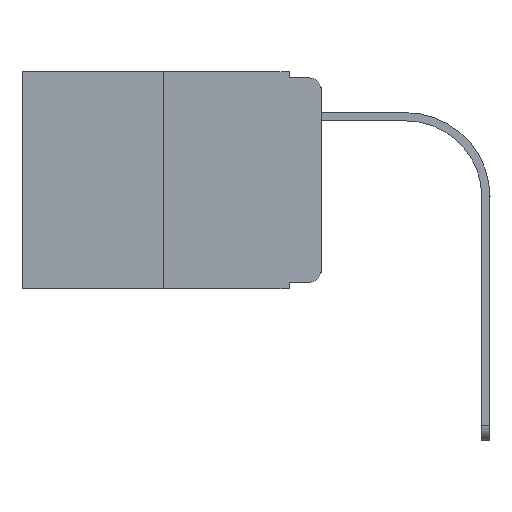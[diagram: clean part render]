
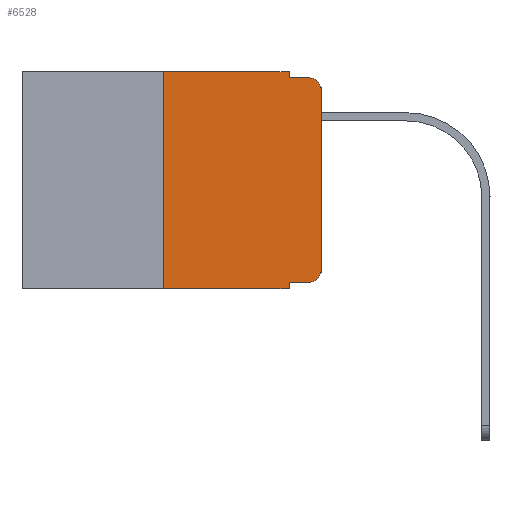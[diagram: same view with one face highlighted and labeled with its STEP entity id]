
A CAD part, left-side view. The second image highlights one B-rep face of the part: STEP entity #6528.
In plain terms, the highlighted planar face has unit normal (-1, 0, 0).
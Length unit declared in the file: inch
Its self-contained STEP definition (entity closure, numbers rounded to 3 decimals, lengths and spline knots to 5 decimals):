
#73 = CARTESIAN_POINT ( 'NONE',  ( 0., 0.051, 0. ) ) ;
#484 = LINE ( 'NONE', #7855, #7972 ) ;
#910 = CARTESIAN_POINT ( 'NONE',  ( 0., 0.25, 0. ) ) ;
#1019 = DIRECTION ( 'NONE',  ( 0., 0., -1. ) ) ;
#1084 = ORIENTED_EDGE ( 'NONE', *, *, #16197, .T. ) ;
#1193 = PLANE ( 'NONE',  #11289 ) ;
#1265 = VECTOR ( 'NONE', #6964, 39.37008 ) ;
#1766 = ORIENTED_EDGE ( 'NONE', *, *, #14694, .F. ) ;
#2194 = VECTOR ( 'NONE', #1019, 39.37008 ) ;
#2731 = VERTEX_POINT ( 'NONE', #16552 ) ;
#2794 = CARTESIAN_POINT ( 'NONE',  ( 0., 0.051, 0. ) ) ;
#3073 = EDGE_CURVE ( 'NONE', #6811, #2731, #14560, .T. ) ;
#3363 = AXIS2_PLACEMENT_3D ( 'NONE', #3949, #7374, #5882 ) ;
#3430 = CARTESIAN_POINT ( 'NONE',  ( 0., 0.473, 0. ) ) ;
#3626 = VECTOR ( 'NONE', #15949, 39.37008 ) ;
#3661 = DIRECTION ( 'NONE',  ( 0., -1., 0. ) ) ;
#3810 = CARTESIAN_POINT ( 'NONE',  ( 0., 0., 0. ) ) ;
#3916 = CARTESIAN_POINT ( 'NONE',  ( 0., 0.473, 0. ) ) ;
#3949 = CARTESIAN_POINT ( 'NONE',  ( 0., 0.02, -0.03 ) ) ;
#4098 = LINE ( 'NONE', #2794, #2194 ) ;
#4325 = DIRECTION ( 'NONE',  ( 0., 0., -1. ) ) ;
#4702 = ORIENTED_EDGE ( 'NONE', *, *, #12635, .T. ) ;
#4916 = LINE ( 'NONE', #3430, #10416 ) ;
#4945 = LINE ( 'NONE', #73, #10716 ) ;
#5126 = EDGE_CURVE ( 'NONE', #10448, #17928, #4098, .T. ) ;
#5464 = CARTESIAN_POINT ( 'NONE',  ( 0., 0.051, -0.01 ) ) ;
#5467 = LINE ( 'NONE', #16133, #7772 ) ;
#5882 = DIRECTION ( 'NONE',  ( 0., 0., -1. ) ) ;
#6190 = ORIENTED_EDGE ( 'NONE', *, *, #16955, .F. ) ;
#6506 = DIRECTION ( 'NONE',  ( 0., -1., 0. ) ) ;
#6528 = ADVANCED_FACE ( 'NONE', ( #8108 ), #1193, .F. ) ;
#6811 = VERTEX_POINT ( 'NONE', #9234 ) ;
#6950 = EDGE_CURVE ( 'NONE', #9740, #12576, #5467, .T. ) ;
#6964 = DIRECTION ( 'NONE',  ( 0., 0., 1. ) ) ;
#7374 = DIRECTION ( 'NONE',  ( -1., 0., 0. ) ) ;
#7514 = CARTESIAN_POINT ( 'NONE',  ( 0., 0.051, -0.343 ) ) ;
#7772 = VECTOR ( 'NONE', #17823, 39.37008 ) ;
#7838 = CIRCLE ( 'NONE', #3363, 0.02 ) ;
#7855 = CARTESIAN_POINT ( 'NONE',  ( 0., 0.051, -0.01 ) ) ;
#7972 = VECTOR ( 'NONE', #3661, 39.37008 ) ;
#8108 = FACE_OUTER_BOUND ( 'NONE', #16885, .T. ) ;
#8746 = DIRECTION ( 'NONE',  ( 0., -1., 0. ) ) ;
#8942 = CARTESIAN_POINT ( 'NONE',  ( 0., 0.051, 0. ) ) ;
#9223 = ORIENTED_EDGE ( 'NONE', *, *, #5126, .F. ) ;
#9234 = CARTESIAN_POINT ( 'NONE',  ( 0., 0.25, -0.343 ) ) ;
#9686 = ORIENTED_EDGE ( 'NONE', *, *, #18891, .T. ) ;
#9688 = ORIENTED_EDGE ( 'NONE', *, *, #3073, .F. ) ;
#9740 = VERTEX_POINT ( 'NONE', #16122 ) ;
#9807 = LINE ( 'NONE', #3810, #3626 ) ;
#10235 = VERTEX_POINT ( 'NONE', #16200 ) ;
#10416 = VECTOR ( 'NONE', #6506, 39.37008 ) ;
#10448 = VERTEX_POINT ( 'NONE', #8942 ) ;
#10490 = VERTEX_POINT ( 'NONE', #7514 ) ;
#10716 = VECTOR ( 'NONE', #13944, 39.37008 ) ;
#11289 = AXIS2_PLACEMENT_3D ( 'NONE', #3916, #11311, #11501 ) ;
#11311 = DIRECTION ( 'NONE',  ( 1., 0., 0. ) ) ;
#11501 = DIRECTION ( 'NONE',  ( 0., 0., -1. ) ) ;
#11631 = CIRCLE ( 'NONE', #12260, 0.02 ) ;
#12260 = AXIS2_PLACEMENT_3D ( 'NONE', #14995, #15186, #4325 ) ;
#12576 = VERTEX_POINT ( 'NONE', #14254 ) ;
#12635 = EDGE_CURVE ( 'NONE', #6811, #10490, #19113, .T. ) ;
#13022 = ORIENTED_EDGE ( 'NONE', *, *, #13123, .T. ) ;
#13123 = EDGE_CURVE ( 'NONE', #16047, #10235, #7838, .T. ) ;
#13944 = DIRECTION ( 'NONE',  ( 0., 0., -1. ) ) ;
#14254 = CARTESIAN_POINT ( 'NONE',  ( 0., 0.02, -0.333 ) ) ;
#14560 = LINE ( 'NONE', #910, #1265 ) ;
#14694 = EDGE_CURVE ( 'NONE', #2731, #10448, #4916, .T. ) ;
#14995 = CARTESIAN_POINT ( 'NONE',  ( 0., 0.02, -0.313 ) ) ;
#15186 = DIRECTION ( 'NONE',  ( -1., 0., 0. ) ) ;
#15365 = EDGE_CURVE ( 'NONE', #9740, #10490, #4945, .T. ) ;
#15423 = ORIENTED_EDGE ( 'NONE', *, *, #6950, .T. ) ;
#15949 = DIRECTION ( 'NONE',  ( 0., 0., 1. ) ) ;
#16047 = VERTEX_POINT ( 'NONE', #16856 ) ;
#16122 = CARTESIAN_POINT ( 'NONE',  ( 0., 0.051, -0.333 ) ) ;
#16133 = CARTESIAN_POINT ( 'NONE',  ( 0., 0.051, -0.333 ) ) ;
#16197 = EDGE_CURVE ( 'NONE', #19112, #16047, #9807, .T. ) ;
#16200 = CARTESIAN_POINT ( 'NONE',  ( 0., 0.02, -0.01 ) ) ;
#16256 = CARTESIAN_POINT ( 'NONE',  ( 0., 0., -0.313 ) ) ;
#16552 = CARTESIAN_POINT ( 'NONE',  ( 0., 0.25, 0. ) ) ;
#16856 = CARTESIAN_POINT ( 'NONE',  ( 0., 0., -0.03 ) ) ;
#16885 = EDGE_LOOP ( 'NONE', ( #1084, #13022, #6190, #9223, #1766, #9688, #4702, #19164, #15423, #9686 ) ) ;
#16955 = EDGE_CURVE ( 'NONE', #17928, #10235, #484, .T. ) ;
#17801 = CARTESIAN_POINT ( 'NONE',  ( 0., 0.473, -0.343 ) ) ;
#17823 = DIRECTION ( 'NONE',  ( 0., -1., 0. ) ) ;
#17928 = VERTEX_POINT ( 'NONE', #5464 ) ;
#18891 = EDGE_CURVE ( 'NONE', #12576, #19112, #11631, .T. ) ;
#19112 = VERTEX_POINT ( 'NONE', #16256 ) ;
#19113 = LINE ( 'NONE', #17801, #19555 ) ;
#19164 = ORIENTED_EDGE ( 'NONE', *, *, #15365, .F. ) ;
#19555 = VECTOR ( 'NONE', #8746, 39.37008 ) ;
